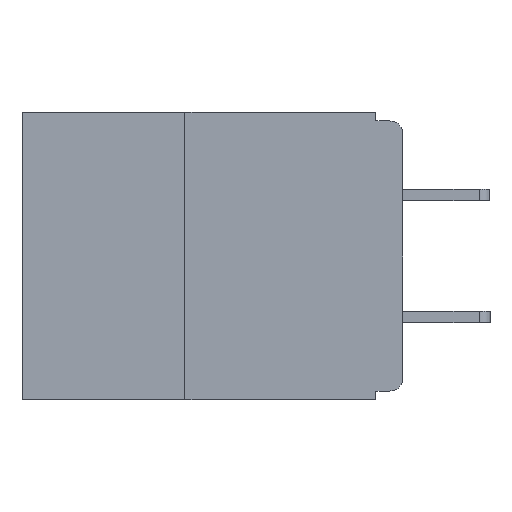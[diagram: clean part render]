
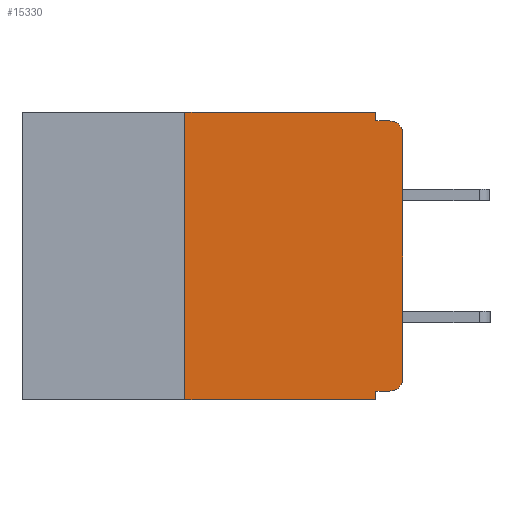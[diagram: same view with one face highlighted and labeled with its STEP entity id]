
A CAD part, left-side view. The second image highlights one B-rep face of the part: STEP entity #15330.
In plain terms, the highlighted planar face has unit normal (-1, 0, 0).
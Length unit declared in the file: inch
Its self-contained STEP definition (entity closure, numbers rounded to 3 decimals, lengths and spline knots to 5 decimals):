
#757 = EDGE_CURVE ( 'NONE', #15381, #10370, #19463, .T. ) ;
#985 = CARTESIAN_POINT ( 'NONE',  ( 0., 0.25, -0.33 ) ) ;
#1775 = EDGE_CURVE ( 'NONE', #15169, #2428, #22148, .T. ) ;
#2046 = VECTOR ( 'NONE', #23064, 39.37008 ) ;
#2204 = EDGE_LOOP ( 'NONE', ( #23162, #23379, #23425, #23783, #23884, #24465, #26318, #26953, #27027, #27791 ) ) ;
#2366 = EDGE_CURVE ( 'NONE', #31123, #8843, #11444, .T. ) ;
#2428 = VERTEX_POINT ( 'NONE', #16253 ) ;
#2600 = AXIS2_PLACEMENT_3D ( 'NONE', #31265, #31190, #31125 ) ;
#3623 = DIRECTION ( 'NONE',  ( 0., 0., 1. ) ) ;
#3755 = EDGE_CURVE ( 'NONE', #30036, #22694, #4167, .T. ) ;
#4167 = CIRCLE ( 'NONE', #2600, 0.015 ) ;
#4884 = CARTESIAN_POINT ( 'NONE',  ( 0., 0., -0.32 ) ) ;
#5467 = CARTESIAN_POINT ( 'NONE',  ( 0., 0.25, 0. ) ) ;
#5942 = DIRECTION ( 'NONE',  ( 0., 0., -1. ) ) ;
#6649 = EDGE_CURVE ( 'NONE', #14273, #21855, #27440, .T. ) ;
#7462 = DIRECTION ( 'NONE',  ( 0., 1., 0. ) ) ;
#7624 = CARTESIAN_POINT ( 'NONE',  ( 0., 0.437, -0.33 ) ) ;
#8009 = CARTESIAN_POINT ( 'NONE',  ( 0., 0., -0.305 ) ) ;
#8182 = DIRECTION ( 'NONE',  ( 0., 0., 1. ) ) ;
#8390 = CARTESIAN_POINT ( 'NONE',  ( 0., 0.25, -0.33 ) ) ;
#8692 = VECTOR ( 'NONE', #27820, 39.37008 ) ;
#8843 = VERTEX_POINT ( 'NONE', #9292 ) ;
#9292 = CARTESIAN_POINT ( 'NONE',  ( 0., 0.015, -0.01 ) ) ;
#9360 = EDGE_CURVE ( 'NONE', #22694, #31123, #18662, .T. ) ;
#9955 = FACE_OUTER_BOUND ( 'NONE', #2204, .T. ) ;
#10370 = VERTEX_POINT ( 'NONE', #5467 ) ;
#10982 = AXIS2_PLACEMENT_3D ( 'NONE', #17762, #17717, #17562 ) ;
#11444 = CIRCLE ( 'NONE', #10982, 0.015 ) ;
#12733 = DIRECTION ( 'NONE',  ( 0., -1., 0. ) ) ;
#13504 = CARTESIAN_POINT ( 'NONE',  ( 0., 0.437, 0. ) ) ;
#14273 = VERTEX_POINT ( 'NONE', #29456 ) ;
#15153 = EDGE_CURVE ( 'NONE', #15381, #21855, #22247, .T. ) ;
#15169 = VERTEX_POINT ( 'NONE', #22930 ) ;
#15330 = ADVANCED_FACE ( 'NONE', ( #9955 ), #18624, .F. ) ;
#15381 = VERTEX_POINT ( 'NONE', #985 ) ;
#15538 = VECTOR ( 'NONE', #12733, 39.37008 ) ;
#15668 = LINE ( 'NONE', #20500, #2046 ) ;
#15678 = VECTOR ( 'NONE', #7462, 39.37008 ) ;
#15736 = DIRECTION ( 'NONE',  ( 0., 0., -1. ) ) ;
#16253 = CARTESIAN_POINT ( 'NONE',  ( 0., 0.031, -0.01 ) ) ;
#16390 = CARTESIAN_POINT ( 'NONE',  ( 0., 0., 0. ) ) ;
#17156 = CARTESIAN_POINT ( 'NONE',  ( 0., 0.031, -0.33 ) ) ;
#17562 = DIRECTION ( 'NONE',  ( 0., 0., -1. ) ) ;
#17717 = DIRECTION ( 'NONE',  ( -1., 0., 0. ) ) ;
#17762 = CARTESIAN_POINT ( 'NONE',  ( 0., 0.015, -0.025 ) ) ;
#18624 = PLANE ( 'NONE',  #30954 ) ;
#18662 = LINE ( 'NONE', #16390, #25307 ) ;
#19207 = DIRECTION ( 'NONE',  ( 0., -1., 0. ) ) ;
#19463 = LINE ( 'NONE', #8390, #31841 ) ;
#19590 = VECTOR ( 'NONE', #19207, 39.37008 ) ;
#20500 = CARTESIAN_POINT ( 'NONE',  ( 0., 0., -0.01 ) ) ;
#21142 = DIRECTION ( 'NONE',  ( 1., 0., 0. ) ) ;
#21581 = LINE ( 'NONE', #4884, #15678 ) ;
#21618 = VECTOR ( 'NONE', #15736, 39.37008 ) ;
#21855 = VERTEX_POINT ( 'NONE', #17156 ) ;
#22097 = EDGE_CURVE ( 'NONE', #2428, #8843, #15668, .T. ) ;
#22148 = LINE ( 'NONE', #27940, #8692 ) ;
#22247 = LINE ( 'NONE', #7624, #15538 ) ;
#22402 = EDGE_CURVE ( 'NONE', #10370, #15169, #26224, .T. ) ;
#22694 = VERTEX_POINT ( 'NONE', #8009 ) ;
#22930 = CARTESIAN_POINT ( 'NONE',  ( 0., 0.031, 0. ) ) ;
#23064 = DIRECTION ( 'NONE',  ( 0., -1., 0. ) ) ;
#23162 = ORIENTED_EDGE ( 'NONE', *, *, #9360, .T. ) ;
#23379 = ORIENTED_EDGE ( 'NONE', *, *, #2366, .T. ) ;
#23425 = ORIENTED_EDGE ( 'NONE', *, *, #22097, .F. ) ;
#23783 = ORIENTED_EDGE ( 'NONE', *, *, #1775, .F. ) ;
#23884 = ORIENTED_EDGE ( 'NONE', *, *, #22402, .F. ) ;
#24465 = ORIENTED_EDGE ( 'NONE', *, *, #757, .F. ) ;
#25307 = VECTOR ( 'NONE', #3623, 39.37008 ) ;
#26224 = LINE ( 'NONE', #29086, #19590 ) ;
#26318 = ORIENTED_EDGE ( 'NONE', *, *, #15153, .T. ) ;
#26953 = ORIENTED_EDGE ( 'NONE', *, *, #6649, .F. ) ;
#27027 = ORIENTED_EDGE ( 'NONE', *, *, #31762, .F. ) ;
#27440 = LINE ( 'NONE', #30628, #21618 ) ;
#27678 = CARTESIAN_POINT ( 'NONE',  ( 0., 0., -0.025 ) ) ;
#27791 = ORIENTED_EDGE ( 'NONE', *, *, #3755, .T. ) ;
#27820 = DIRECTION ( 'NONE',  ( 0., 0., -1. ) ) ;
#27940 = CARTESIAN_POINT ( 'NONE',  ( 0., 0.031, 0. ) ) ;
#29086 = CARTESIAN_POINT ( 'NONE',  ( 0., 0.437, 0. ) ) ;
#29456 = CARTESIAN_POINT ( 'NONE',  ( 0., 0.031, -0.32 ) ) ;
#30036 = VERTEX_POINT ( 'NONE', #30607 ) ;
#30607 = CARTESIAN_POINT ( 'NONE',  ( 0., 0.015, -0.32 ) ) ;
#30628 = CARTESIAN_POINT ( 'NONE',  ( 0., 0.031, -0.33 ) ) ;
#30954 = AXIS2_PLACEMENT_3D ( 'NONE', #13504, #21142, #5942 ) ;
#31123 = VERTEX_POINT ( 'NONE', #27678 ) ;
#31125 = DIRECTION ( 'NONE',  ( 0., 0., -1. ) ) ;
#31190 = DIRECTION ( 'NONE',  ( -1., 0., 0. ) ) ;
#31265 = CARTESIAN_POINT ( 'NONE',  ( 0., 0.015, -0.305 ) ) ;
#31762 = EDGE_CURVE ( 'NONE', #30036, #14273, #21581, .T. ) ;
#31841 = VECTOR ( 'NONE', #8182, 39.37008 ) ;
